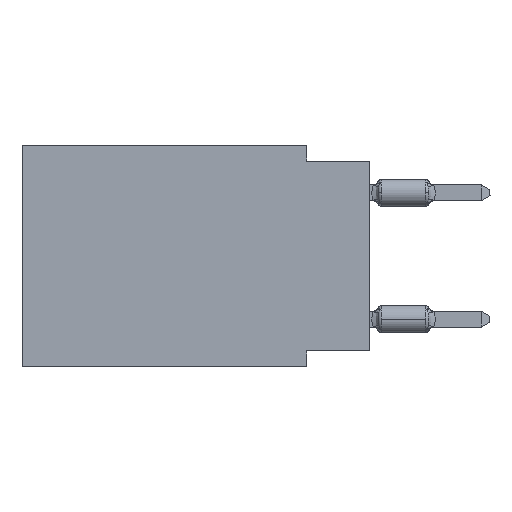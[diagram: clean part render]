
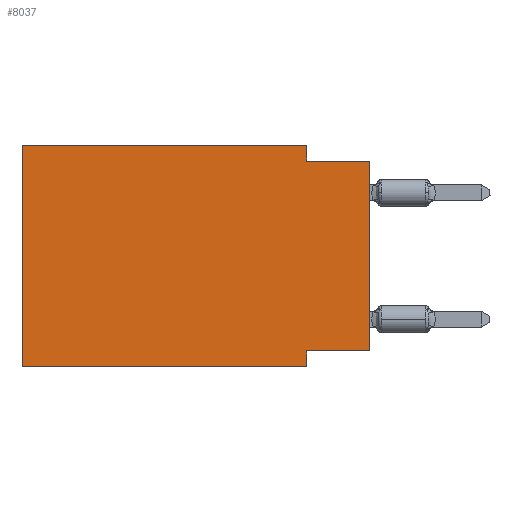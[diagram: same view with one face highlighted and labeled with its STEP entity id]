
A CAD part, left-side view. The second image highlights one B-rep face of the part: STEP entity #8037.
In plain terms, the highlighted planar face has unit normal (-1, 0, 0).
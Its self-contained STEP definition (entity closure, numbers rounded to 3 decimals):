
#342 = CARTESIAN_POINT ( 'NONE',  ( 0., 0., -0.635 ) ) ;
#963 = CARTESIAN_POINT ( 'NONE',  ( 0., 2.54, -0.635 ) ) ;
#2082 = DIRECTION ( 'NONE',  ( 0., -1., 0. ) ) ;
#3399 = VERTEX_POINT ( 'NONE', #11831 ) ;
#3709 = DIRECTION ( 'NONE',  ( 0., 0., 1. ) ) ;
#3847 = DIRECTION ( 'NONE',  ( 0., -1., 0. ) ) ;
#5296 = DIRECTION ( 'NONE',  ( 0., 0., -1. ) ) ;
#5520 = CARTESIAN_POINT ( 'NONE',  ( 0., 0., -8.255 ) ) ;
#5534 = LINE ( 'NONE', #5990, #25135 ) ;
#5990 = CARTESIAN_POINT ( 'NONE',  ( 0., 0., -0.635 ) ) ;
#6005 = EDGE_CURVE ( 'NONE', #30375, #8130, #8133, .T. ) ;
#6008 = ORIENTED_EDGE ( 'NONE', *, *, #19560, .F. ) ;
#6952 = EDGE_CURVE ( 'NONE', #9947, #16186, #30046, .T. ) ;
#7158 = CARTESIAN_POINT ( 'NONE',  ( 0., 2.54, -8.89 ) ) ;
#7351 = LINE ( 'NONE', #28153, #27468 ) ;
#7614 = CARTESIAN_POINT ( 'NONE',  ( 0., 13.97, 0. ) ) ;
#7986 = CARTESIAN_POINT ( 'NONE',  ( 0., 2.54, 0. ) ) ;
#8037 = ADVANCED_FACE ( 'NONE', ( #19801 ), #21944, .F. ) ;
#8074 = ORIENTED_EDGE ( 'NONE', *, *, #6005, .F. ) ;
#8130 = VERTEX_POINT ( 'NONE', #963 ) ;
#8133 = LINE ( 'NONE', #7986, #22505 ) ;
#8429 = VERTEX_POINT ( 'NONE', #13902 ) ;
#9489 = VECTOR ( 'NONE', #3709, 1000. ) ;
#9947 = VERTEX_POINT ( 'NONE', #15114 ) ;
#10793 = EDGE_CURVE ( 'NONE', #8429, #16186, #14847, .T. ) ;
#11335 = LINE ( 'NONE', #20765, #19394 ) ;
#11416 = ORIENTED_EDGE ( 'NONE', *, *, #14604, .T. ) ;
#11747 = EDGE_CURVE ( 'NONE', #8130, #17326, #5534, .T. ) ;
#11831 = CARTESIAN_POINT ( 'NONE',  ( 0., 13.97, 0. ) ) ;
#11860 = ORIENTED_EDGE ( 'NONE', *, *, #10793, .F. ) ;
#12163 = ORIENTED_EDGE ( 'NONE', *, *, #6952, .T. ) ;
#12483 = EDGE_LOOP ( 'NONE', ( #11416, #26847, #8074, #6008, #27425, #12163, #11860, #14046 ) ) ;
#13902 = CARTESIAN_POINT ( 'NONE',  ( 0., 2.54, -8.255 ) ) ;
#14046 = ORIENTED_EDGE ( 'NONE', *, *, #24474, .F. ) ;
#14604 = EDGE_CURVE ( 'NONE', #22944, #17326, #26995, .T. ) ;
#14847 = LINE ( 'NONE', #7158, #27551 ) ;
#15114 = CARTESIAN_POINT ( 'NONE',  ( 0., 13.97, -8.89 ) ) ;
#16186 = VERTEX_POINT ( 'NONE', #19595 ) ;
#16747 = DIRECTION ( 'NONE',  ( 0., 1., 0. ) ) ;
#17326 = VERTEX_POINT ( 'NONE', #342 ) ;
#19067 = AXIS2_PLACEMENT_3D ( 'NONE', #7614, #19646, #5296 ) ;
#19371 = LINE ( 'NONE', #21693, #29923 ) ;
#19394 = VECTOR ( 'NONE', #2082, 1000. ) ;
#19560 = EDGE_CURVE ( 'NONE', #3399, #30375, #11335, .T. ) ;
#19595 = CARTESIAN_POINT ( 'NONE',  ( 0., 2.54, -8.89 ) ) ;
#19646 = DIRECTION ( 'NONE',  ( 1., 0., 0. ) ) ;
#19801 = FACE_OUTER_BOUND ( 'NONE', #12483, .T. ) ;
#20765 = CARTESIAN_POINT ( 'NONE',  ( 0., 13.97, 0. ) ) ;
#21693 = CARTESIAN_POINT ( 'NONE',  ( 0., 13.97, 0. ) ) ;
#21759 = CARTESIAN_POINT ( 'NONE',  ( 0., 2.54, 0. ) ) ;
#21944 = PLANE ( 'NONE',  #19067 ) ;
#22505 = VECTOR ( 'NONE', #26775, 1000. ) ;
#22944 = VERTEX_POINT ( 'NONE', #5520 ) ;
#23985 = DIRECTION ( 'NONE',  ( 0., 0., 1. ) ) ;
#24474 = EDGE_CURVE ( 'NONE', #22944, #8429, #7351, .T. ) ;
#24575 = EDGE_CURVE ( 'NONE', #9947, #3399, #19371, .T. ) ;
#24789 = DIRECTION ( 'NONE',  ( 0., -1., 0. ) ) ;
#24975 = CARTESIAN_POINT ( 'NONE',  ( 0., 13.97, -8.89 ) ) ;
#25135 = VECTOR ( 'NONE', #24789, 1000. ) ;
#26255 = DIRECTION ( 'NONE',  ( 0., 0., -1. ) ) ;
#26775 = DIRECTION ( 'NONE',  ( 0., 0., -1. ) ) ;
#26847 = ORIENTED_EDGE ( 'NONE', *, *, #11747, .F. ) ;
#26995 = LINE ( 'NONE', #27151, #9489 ) ;
#27151 = CARTESIAN_POINT ( 'NONE',  ( 0., 0., 0. ) ) ;
#27425 = ORIENTED_EDGE ( 'NONE', *, *, #24575, .F. ) ;
#27468 = VECTOR ( 'NONE', #16747, 1000. ) ;
#27551 = VECTOR ( 'NONE', #26255, 1000. ) ;
#28153 = CARTESIAN_POINT ( 'NONE',  ( 0., 0., -8.255 ) ) ;
#29923 = VECTOR ( 'NONE', #23985, 1000. ) ;
#30046 = LINE ( 'NONE', #24975, #30404 ) ;
#30375 = VERTEX_POINT ( 'NONE', #21759 ) ;
#30404 = VECTOR ( 'NONE', #3847, 1000. ) ;
